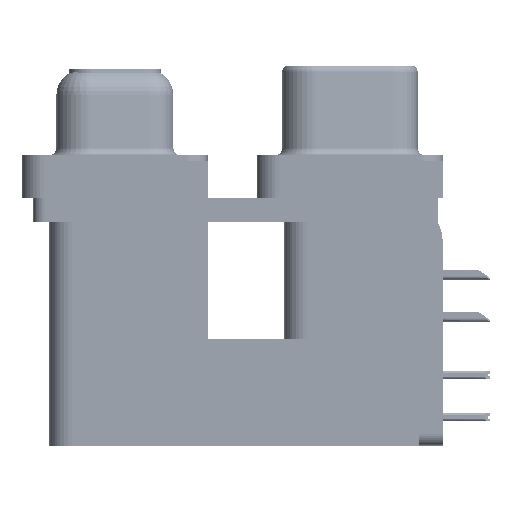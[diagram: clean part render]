
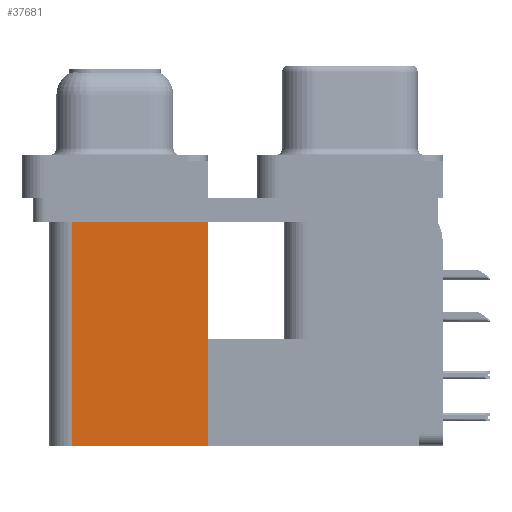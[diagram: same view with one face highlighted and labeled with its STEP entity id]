
A CAD part, left-side view. The second image highlights one B-rep face of the part: STEP entity #37681.
In plain terms, the highlighted planar face has unit normal (-1, 0, 0).
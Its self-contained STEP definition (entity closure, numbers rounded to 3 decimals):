
#549 = EDGE_CURVE ( 'NONE', #48158, #30788, #28316, .T. ) ;
#2580 = DIRECTION ( 'NONE',  ( 0., 1., 0. ) ) ;
#2762 = VECTOR ( 'NONE', #54726, 1000. ) ;
#3912 = DIRECTION ( 'NONE',  ( 0., 1., 0. ) ) ;
#9958 = LINE ( 'NONE', #20519, #46045 ) ;
#11098 = VERTEX_POINT ( 'NONE', #27528 ) ;
#13879 = ORIENTED_EDGE ( 'NONE', *, *, #54216, .T. ) ;
#20519 = CARTESIAN_POINT ( 'NONE',  ( 3.79, 18.8, -19.2 ) ) ;
#23571 = DIRECTION ( 'NONE',  ( 0., 1., 0. ) ) ;
#24711 = CARTESIAN_POINT ( 'NONE',  ( 3.79, 9.6, -2.5 ) ) ;
#25513 = ORIENTED_EDGE ( 'NONE', *, *, #549, .F. ) ;
#27528 = CARTESIAN_POINT ( 'NONE',  ( 3.79, 18.8, -2.5 ) ) ;
#28316 = LINE ( 'NONE', #47457, #34826 ) ;
#28669 = EDGE_CURVE ( 'NONE', #30788, #11098, #9958, .T. ) ;
#30788 = VERTEX_POINT ( 'NONE', #57749 ) ;
#34826 = VECTOR ( 'NONE', #2580, 1000. ) ;
#35682 = DIRECTION ( 'NONE',  ( 0., 0., 1. ) ) ;
#37681 = ADVANCED_FACE ( 'NONE', ( #58879 ), #43035, .F. ) ;
#38057 = EDGE_CURVE ( 'NONE', #48158, #57836, #47502, .T. ) ;
#40220 = CARTESIAN_POINT ( 'NONE',  ( 3.79, 9.6, -19.2 ) ) ;
#41217 = ORIENTED_EDGE ( 'NONE', *, *, #28669, .F. ) ;
#43035 = PLANE ( 'NONE',  #51173 ) ;
#43668 = DIRECTION ( 'NONE',  ( 1., 0., 0. ) ) ;
#44169 = CARTESIAN_POINT ( 'NONE',  ( 3.79, 9.6, -19.2 ) ) ;
#46011 = EDGE_LOOP ( 'NONE', ( #13879, #41217, #25513, #47012 ) ) ;
#46045 = VECTOR ( 'NONE', #35682, 1000. ) ;
#47012 = ORIENTED_EDGE ( 'NONE', *, *, #38057, .T. ) ;
#47457 = CARTESIAN_POINT ( 'NONE',  ( 3.79, 9.6, -19.2 ) ) ;
#47502 = LINE ( 'NONE', #44169, #2762 ) ;
#48158 = VERTEX_POINT ( 'NONE', #40220 ) ;
#48801 = LINE ( 'NONE', #24711, #52286 ) ;
#51173 = AXIS2_PLACEMENT_3D ( 'NONE', #54228, #43668, #23571 ) ;
#52286 = VECTOR ( 'NONE', #3912, 1000. ) ;
#52883 = CARTESIAN_POINT ( 'NONE',  ( 3.79, 9.6, -2.5 ) ) ;
#54216 = EDGE_CURVE ( 'NONE', #57836, #11098, #48801, .T. ) ;
#54228 = CARTESIAN_POINT ( 'NONE',  ( 3.79, 9.6, -19.2 ) ) ;
#54726 = DIRECTION ( 'NONE',  ( 0., 0., 1. ) ) ;
#57749 = CARTESIAN_POINT ( 'NONE',  ( 3.79, 18.8, -19.2 ) ) ;
#57836 = VERTEX_POINT ( 'NONE', #52883 ) ;
#58879 = FACE_OUTER_BOUND ( 'NONE', #46011, .T. ) ;
